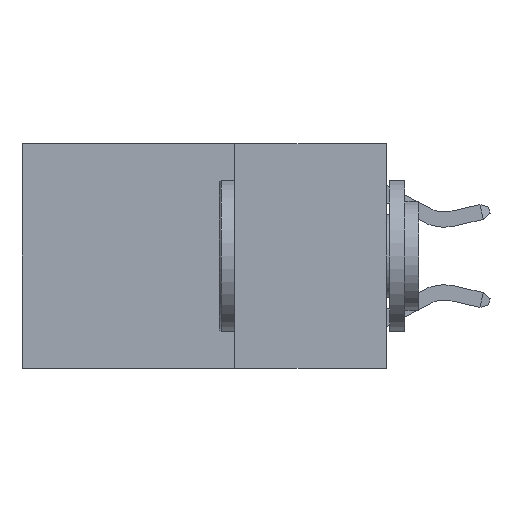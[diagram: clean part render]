
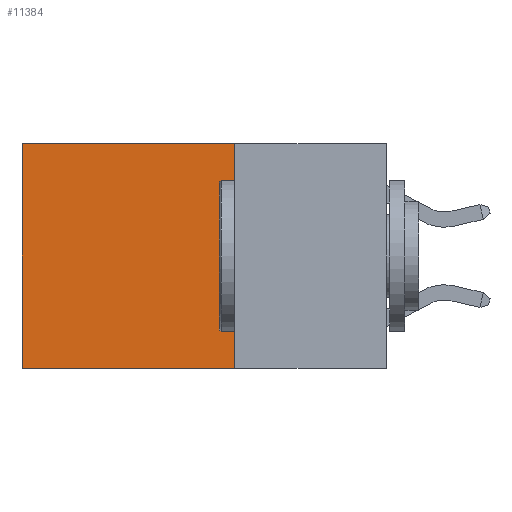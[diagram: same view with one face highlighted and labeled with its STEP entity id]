
A CAD part, left-side view. The second image highlights one B-rep face of the part: STEP entity #11384.
In plain terms, the highlighted planar face has unit normal (-1, 0, 0).
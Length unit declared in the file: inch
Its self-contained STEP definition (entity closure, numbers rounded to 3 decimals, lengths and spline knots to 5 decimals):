
#178 = VERTEX_POINT ( 'NONE', #8277 ) ;
#896 = VECTOR ( 'NONE', #8710, 39.37008 ) ;
#1265 = CARTESIAN_POINT ( 'NONE',  ( 0.2625, 0.25, 0. ) ) ;
#1715 = CARTESIAN_POINT ( 'NONE',  ( 0.2625, 0.25, -0.37 ) ) ;
#2205 = CARTESIAN_POINT ( 'NONE',  ( 0.2625, 0.6, 0. ) ) ;
#2233 = VERTEX_POINT ( 'NONE', #12120 ) ;
#2756 = CARTESIAN_POINT ( 'NONE',  ( 0.2625, 0.25, -0.37 ) ) ;
#2974 = VERTEX_POINT ( 'NONE', #2756 ) ;
#3298 = AXIS2_PLACEMENT_3D ( 'NONE', #10690, #4468, #9201 ) ;
#4107 = ORIENTED_EDGE ( 'NONE', *, *, #7653, .T. ) ;
#4468 = DIRECTION ( 'NONE',  ( 1., 0., 0. ) ) ;
#4762 = FACE_OUTER_BOUND ( 'NONE', #10947, .T. ) ;
#5797 = DIRECTION ( 'NONE',  ( 0., 0., -1. ) ) ;
#5989 = PLANE ( 'NONE',  #3298 ) ;
#6196 = ORIENTED_EDGE ( 'NONE', *, *, #9670, .T. ) ;
#7417 = VERTEX_POINT ( 'NONE', #2205 ) ;
#7580 = ORIENTED_EDGE ( 'NONE', *, *, #13410, .F. ) ;
#7653 = EDGE_CURVE ( 'NONE', #178, #7417, #8558, .T. ) ;
#8277 = CARTESIAN_POINT ( 'NONE',  ( 0.2625, 0.25, 0. ) ) ;
#8558 = LINE ( 'NONE', #1265, #14239 ) ;
#8710 = DIRECTION ( 'NONE',  ( 0., 0., -1. ) ) ;
#9201 = DIRECTION ( 'NONE',  ( 0., 0., -1. ) ) ;
#9644 = CARTESIAN_POINT ( 'NONE',  ( 0.2625, 0.25, 0. ) ) ;
#9670 = EDGE_CURVE ( 'NONE', #7417, #2233, #12072, .T. ) ;
#9911 = LINE ( 'NONE', #1715, #12902 ) ;
#10535 = DIRECTION ( 'NONE',  ( 0., 1., 0. ) ) ;
#10690 = CARTESIAN_POINT ( 'NONE',  ( 0.2625, 0.25, 0. ) ) ;
#10947 = EDGE_LOOP ( 'NONE', ( #6196, #7580, #13798, #4107 ) ) ;
#11384 = ADVANCED_FACE ( 'NONE', ( #4762 ), #5989, .F. ) ;
#11586 = CARTESIAN_POINT ( 'NONE',  ( 0.2625, 0.6, 0. ) ) ;
#12072 = LINE ( 'NONE', #11586, #12859 ) ;
#12120 = CARTESIAN_POINT ( 'NONE',  ( 0.2625, 0.6, -0.37 ) ) ;
#12859 = VECTOR ( 'NONE', #5797, 39.37008 ) ;
#12902 = VECTOR ( 'NONE', #13686, 39.37008 ) ;
#13410 = EDGE_CURVE ( 'NONE', #2974, #2233, #9911, .T. ) ;
#13686 = DIRECTION ( 'NONE',  ( 0., 1., 0. ) ) ;
#13798 = ORIENTED_EDGE ( 'NONE', *, *, #15104, .F. ) ;
#14239 = VECTOR ( 'NONE', #10535, 39.37008 ) ;
#14558 = LINE ( 'NONE', #9644, #896 ) ;
#15104 = EDGE_CURVE ( 'NONE', #178, #2974, #14558, .T. ) ;
